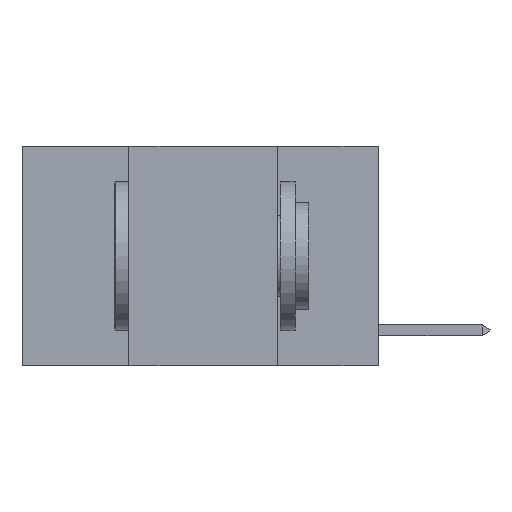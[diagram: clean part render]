
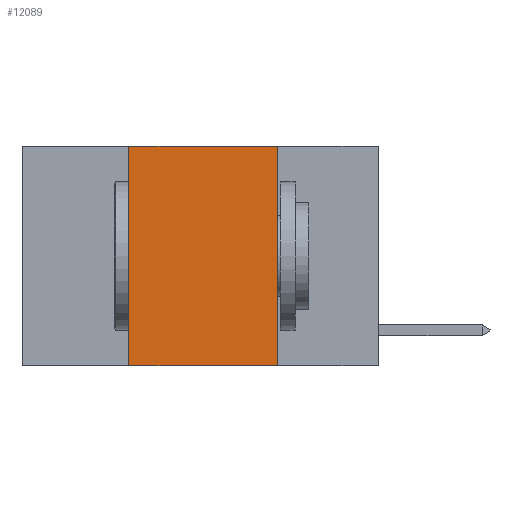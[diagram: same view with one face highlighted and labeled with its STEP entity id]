
A CAD part, left-side view. The second image highlights one B-rep face of the part: STEP entity #12089.
In plain terms, the highlighted planar face has unit normal (-1, 0, 0).
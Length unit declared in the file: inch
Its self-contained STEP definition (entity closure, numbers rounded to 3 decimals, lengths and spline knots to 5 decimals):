
#171 = EDGE_CURVE ( 'NONE', #17760, #14178, #22443, .T. ) ;
#724 = DIRECTION ( 'NONE',  ( 0., 0., -1. ) ) ;
#1233 = ORIENTED_EDGE ( 'NONE', *, *, #4259, .F. ) ;
#1836 = CARTESIAN_POINT ( 'NONE',  ( 0., 0.42, 0. ) ) ;
#2221 = VERTEX_POINT ( 'NONE', #1836 ) ;
#2406 = LINE ( 'NONE', #6092, #10062 ) ;
#2602 = CARTESIAN_POINT ( 'NONE',  ( 0., 0.6, 0. ) ) ;
#2642 = DIRECTION ( 'NONE',  ( 0., -1., 0. ) ) ;
#3201 = CARTESIAN_POINT ( 'NONE',  ( 0., 0.17, -0.37 ) ) ;
#3973 = VECTOR ( 'NONE', #12393, 39.37008 ) ;
#4259 = EDGE_CURVE ( 'NONE', #17760, #2221, #15806, .T. ) ;
#4735 = CARTESIAN_POINT ( 'NONE',  ( 0., 0.6, -0.37 ) ) ;
#5923 = DIRECTION ( 'NONE',  ( 0., 0., -1. ) ) ;
#6092 = CARTESIAN_POINT ( 'NONE',  ( 0., 0.6, 0. ) ) ;
#6415 = FACE_OUTER_BOUND ( 'NONE', #7516, .T. ) ;
#6892 = CARTESIAN_POINT ( 'NONE',  ( 0., 0.17, 0. ) ) ;
#7516 = EDGE_LOOP ( 'NONE', ( #10378, #24885, #1233, #18488 ) ) ;
#8420 = EDGE_CURVE ( 'NONE', #13580, #14178, #18985, .T. ) ;
#8985 = CARTESIAN_POINT ( 'NONE',  ( 0., 0.17, 0. ) ) ;
#10062 = VECTOR ( 'NONE', #2642, 39.37008 ) ;
#10294 = DIRECTION ( 'NONE',  ( 1., 0., 0. ) ) ;
#10378 = ORIENTED_EDGE ( 'NONE', *, *, #8420, .F. ) ;
#11997 = CARTESIAN_POINT ( 'NONE',  ( 0., 0.42, 0. ) ) ;
#12089 = ADVANCED_FACE ( 'NONE', ( #6415 ), #14040, .F. ) ;
#12249 = AXIS2_PLACEMENT_3D ( 'NONE', #2602, #10294, #724 ) ;
#12393 = DIRECTION ( 'NONE',  ( 0., -1., 0. ) ) ;
#13580 = VERTEX_POINT ( 'NONE', #8985 ) ;
#14040 = PLANE ( 'NONE',  #12249 ) ;
#14178 = VERTEX_POINT ( 'NONE', #3201 ) ;
#15806 = LINE ( 'NONE', #11997, #23986 ) ;
#16162 = VECTOR ( 'NONE', #5923, 39.37008 ) ;
#17497 = DIRECTION ( 'NONE',  ( 0., 0., 1. ) ) ;
#17760 = VERTEX_POINT ( 'NONE', #22269 ) ;
#18488 = ORIENTED_EDGE ( 'NONE', *, *, #171, .T. ) ;
#18985 = LINE ( 'NONE', #6892, #16162 ) ;
#22269 = CARTESIAN_POINT ( 'NONE',  ( 0., 0.42, -0.37 ) ) ;
#22443 = LINE ( 'NONE', #4735, #3973 ) ;
#23812 = EDGE_CURVE ( 'NONE', #2221, #13580, #2406, .T. ) ;
#23986 = VECTOR ( 'NONE', #17497, 39.37008 ) ;
#24885 = ORIENTED_EDGE ( 'NONE', *, *, #23812, .F. ) ;
